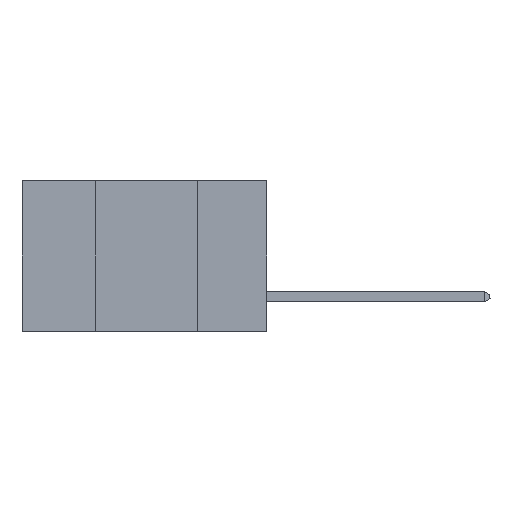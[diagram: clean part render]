
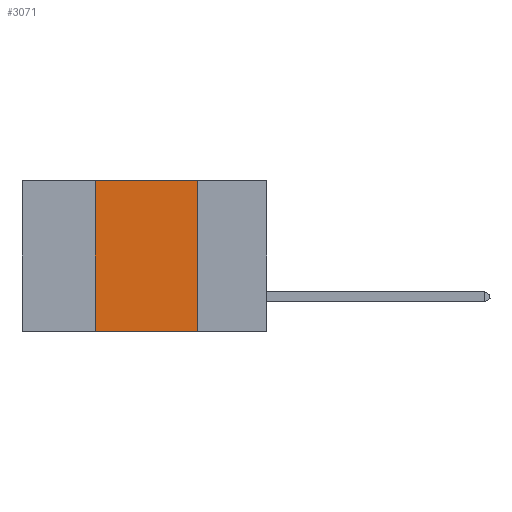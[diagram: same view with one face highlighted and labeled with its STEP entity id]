
A CAD part, left-side view. The second image highlights one B-rep face of the part: STEP entity #3071.
In plain terms, the highlighted planar face has unit normal (-1, 0, 0).
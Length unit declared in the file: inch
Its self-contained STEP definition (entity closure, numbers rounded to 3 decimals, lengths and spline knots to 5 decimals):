
#24 = VECTOR ( 'NONE', #4590, 39.37008 ) ;
#591 = CARTESIAN_POINT ( 'NONE',  ( 0., 0.17, 0. ) ) ;
#660 = EDGE_CURVE ( 'NONE', #10883, #9434, #2524, .T. ) ;
#1032 = EDGE_LOOP ( 'NONE', ( #12329, #11982, #1841, #5889 ) ) ;
#1197 = PLANE ( 'NONE',  #6893 ) ;
#1479 = VECTOR ( 'NONE', #4675, 39.37008 ) ;
#1841 = ORIENTED_EDGE ( 'NONE', *, *, #6246, .F. ) ;
#1957 = VECTOR ( 'NONE', #12367, 39.37008 ) ;
#2370 = CARTESIAN_POINT ( 'NONE',  ( 0., 0.17, 0. ) ) ;
#2467 = EDGE_CURVE ( 'NONE', #9434, #12266, #12058, .T. ) ;
#2524 = LINE ( 'NONE', #8572, #1479 ) ;
#3071 = ADVANCED_FACE ( 'NONE', ( #5379 ), #1197, .F. ) ;
#3559 = VECTOR ( 'NONE', #7292, 39.37008 ) ;
#4100 = LINE ( 'NONE', #6754, #1957 ) ;
#4590 = DIRECTION ( 'NONE',  ( 0., -1., 0. ) ) ;
#4675 = DIRECTION ( 'NONE',  ( 0., -1., 0. ) ) ;
#5129 = EDGE_CURVE ( 'NONE', #11621, #12266, #10963, .T. ) ;
#5379 = FACE_OUTER_BOUND ( 'NONE', #1032, .T. ) ;
#5889 = ORIENTED_EDGE ( 'NONE', *, *, #5129, .T. ) ;
#6246 = EDGE_CURVE ( 'NONE', #11621, #10883, #4100, .T. ) ;
#6754 = CARTESIAN_POINT ( 'NONE',  ( 0., 0.42, 0. ) ) ;
#6893 = AXIS2_PLACEMENT_3D ( 'NONE', #7968, #9057, #10037 ) ;
#7292 = DIRECTION ( 'NONE',  ( 0., 0., -1. ) ) ;
#7803 = CARTESIAN_POINT ( 'NONE',  ( 0., 0.17, -0.37 ) ) ;
#7968 = CARTESIAN_POINT ( 'NONE',  ( 0., 0.6, 0. ) ) ;
#8572 = CARTESIAN_POINT ( 'NONE',  ( 0., 0.6, 0. ) ) ;
#9057 = DIRECTION ( 'NONE',  ( 1., 0., 0. ) ) ;
#9434 = VERTEX_POINT ( 'NONE', #591 ) ;
#10037 = DIRECTION ( 'NONE',  ( 0., 0., -1. ) ) ;
#10528 = CARTESIAN_POINT ( 'NONE',  ( 0., 0.42, -0.37 ) ) ;
#10883 = VERTEX_POINT ( 'NONE', #12338 ) ;
#10963 = LINE ( 'NONE', #12246, #24 ) ;
#11621 = VERTEX_POINT ( 'NONE', #10528 ) ;
#11982 = ORIENTED_EDGE ( 'NONE', *, *, #660, .F. ) ;
#12058 = LINE ( 'NONE', #2370, #3559 ) ;
#12246 = CARTESIAN_POINT ( 'NONE',  ( 0., 0.6, -0.37 ) ) ;
#12266 = VERTEX_POINT ( 'NONE', #7803 ) ;
#12329 = ORIENTED_EDGE ( 'NONE', *, *, #2467, .F. ) ;
#12338 = CARTESIAN_POINT ( 'NONE',  ( 0., 0.42, 0. ) ) ;
#12367 = DIRECTION ( 'NONE',  ( 0., 0., 1. ) ) ;
